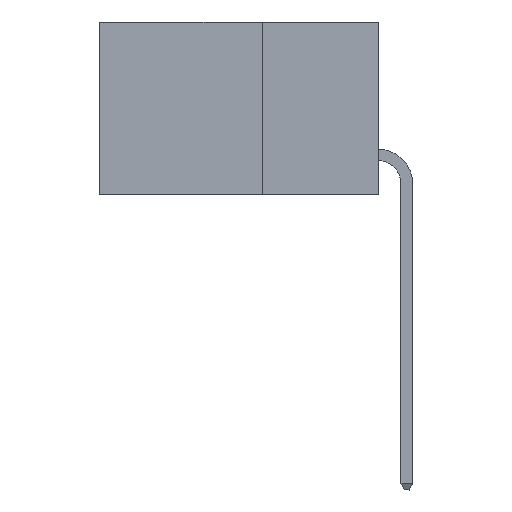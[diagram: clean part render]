
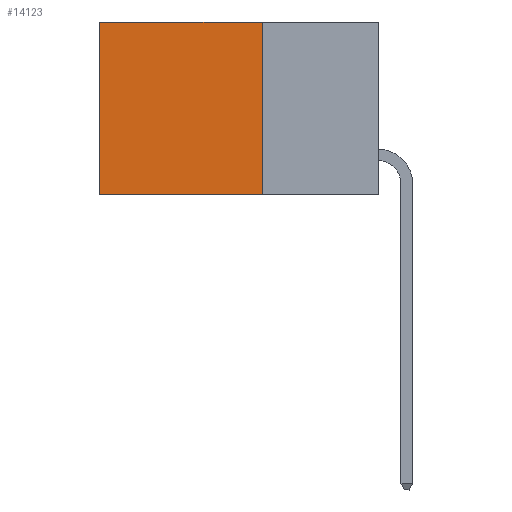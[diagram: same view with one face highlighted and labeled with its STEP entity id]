
A CAD part, left-side view. The second image highlights one B-rep face of the part: STEP entity #14123.
In plain terms, the highlighted planar face has unit normal (-1, 0, 0).
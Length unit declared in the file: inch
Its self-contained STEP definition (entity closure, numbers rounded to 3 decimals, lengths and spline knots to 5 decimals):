
#1351 = FACE_OUTER_BOUND ( 'NONE', #9236, .T. ) ;
#1814 = PLANE ( 'NONE',  #16514 ) ;
#1892 = LINE ( 'NONE', #3431, #17982 ) ;
#2208 = ORIENTED_EDGE ( 'NONE', *, *, #7760, .F. ) ;
#3110 = EDGE_CURVE ( 'NONE', #18939, #4223, #12577, .T. ) ;
#3318 = VECTOR ( 'NONE', #15575, 39.37008 ) ;
#3431 = CARTESIAN_POINT ( 'NONE',  ( 0.298, 0.25, -0.37 ) ) ;
#3830 = VERTEX_POINT ( 'NONE', #19043 ) ;
#3958 = ORIENTED_EDGE ( 'NONE', *, *, #6347, .F. ) ;
#4223 = VERTEX_POINT ( 'NONE', #4414 ) ;
#4414 = CARTESIAN_POINT ( 'NONE',  ( 0.298, 0.6, -0.37 ) ) ;
#4988 = DIRECTION ( 'NONE',  ( 0., 0., -1. ) ) ;
#4996 = CARTESIAN_POINT ( 'NONE',  ( 0.298, 0.6, 0. ) ) ;
#5014 = DIRECTION ( 'NONE',  ( 0., 1., 0. ) ) ;
#5252 = VECTOR ( 'NONE', #9701, 39.37008 ) ;
#5261 = VERTEX_POINT ( 'NONE', #13131 ) ;
#5626 = CARTESIAN_POINT ( 'NONE',  ( 0.298, 0.6, 0. ) ) ;
#6347 = EDGE_CURVE ( 'NONE', #5261, #4223, #1892, .T. ) ;
#7760 = EDGE_CURVE ( 'NONE', #3830, #5261, #13991, .T. ) ;
#7975 = VECTOR ( 'NONE', #12725, 39.37008 ) ;
#8146 = CARTESIAN_POINT ( 'NONE',  ( 0.298, 0.25, 0. ) ) ;
#9236 = EDGE_LOOP ( 'NONE', ( #10923, #3958, #2208, #12921 ) ) ;
#9701 = DIRECTION ( 'NONE',  ( 0., 0., -1. ) ) ;
#10923 = ORIENTED_EDGE ( 'NONE', *, *, #3110, .T. ) ;
#11590 = LINE ( 'NONE', #14004, #3318 ) ;
#12577 = LINE ( 'NONE', #4996, #7975 ) ;
#12721 = CARTESIAN_POINT ( 'NONE',  ( 0.298, 0.25, 0. ) ) ;
#12725 = DIRECTION ( 'NONE',  ( 0., 0., -1. ) ) ;
#12921 = ORIENTED_EDGE ( 'NONE', *, *, #13986, .T. ) ;
#13131 = CARTESIAN_POINT ( 'NONE',  ( 0.298, 0.25, -0.37 ) ) ;
#13986 = EDGE_CURVE ( 'NONE', #3830, #18939, #11590, .T. ) ;
#13991 = LINE ( 'NONE', #8146, #5252 ) ;
#14004 = CARTESIAN_POINT ( 'NONE',  ( 0.298, 0.25, 0. ) ) ;
#14123 = ADVANCED_FACE ( 'NONE', ( #1351 ), #1814, .F. ) ;
#14272 = DIRECTION ( 'NONE',  ( 1., 0., 0. ) ) ;
#15575 = DIRECTION ( 'NONE',  ( 0., 1., 0. ) ) ;
#16514 = AXIS2_PLACEMENT_3D ( 'NONE', #12721, #14272, #4988 ) ;
#17982 = VECTOR ( 'NONE', #5014, 39.37008 ) ;
#18939 = VERTEX_POINT ( 'NONE', #5626 ) ;
#19043 = CARTESIAN_POINT ( 'NONE',  ( 0.298, 0.25, 0. ) ) ;
